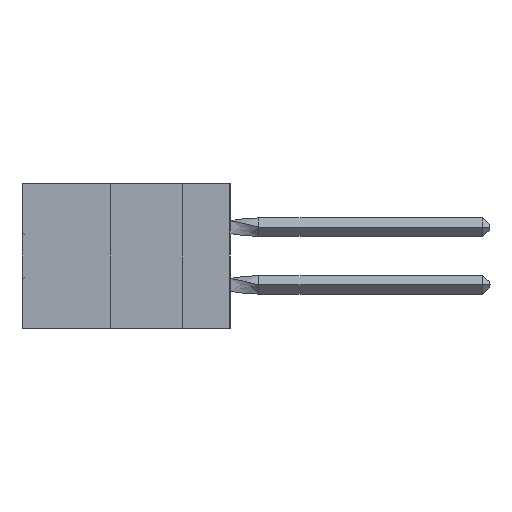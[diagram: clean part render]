
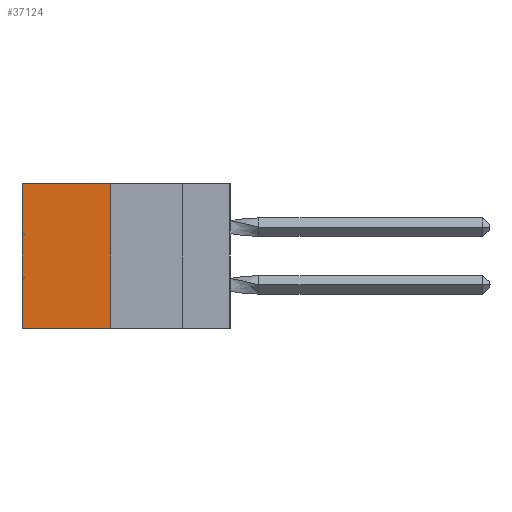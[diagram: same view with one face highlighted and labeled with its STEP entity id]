
A CAD part, left-side view. The second image highlights one B-rep face of the part: STEP entity #37124.
In plain terms, the highlighted planar face has unit normal (-1, 0, 0).
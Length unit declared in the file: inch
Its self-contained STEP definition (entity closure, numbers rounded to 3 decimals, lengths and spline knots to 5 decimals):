
#1311 = DIRECTION ( 'NONE',  ( 0., 0., -1. ) ) ;
#5220 = VERTEX_POINT ( 'NONE', #35647 ) ;
#5736 = FACE_OUTER_BOUND ( 'NONE', #34759, .T. ) ;
#5968 = ORIENTED_EDGE ( 'NONE', *, *, #28280, .T. ) ;
#6668 = VERTEX_POINT ( 'NONE', #11920 ) ;
#7921 = CARTESIAN_POINT ( 'NONE',  ( 0.305, 0.413, 0. ) ) ;
#8298 = EDGE_CURVE ( 'NONE', #5220, #6668, #28618, .T. ) ;
#9250 = DIRECTION ( 'NONE',  ( 0., 1., 0. ) ) ;
#10752 = VERTEX_POINT ( 'NONE', #39555 ) ;
#11899 = CARTESIAN_POINT ( 'NONE',  ( 0.305, 0.413, -0.5 ) ) ;
#11920 = CARTESIAN_POINT ( 'NONE',  ( 0.305, 0.413, -0.5 ) ) ;
#13196 = ORIENTED_EDGE ( 'NONE', *, *, #34501, .T. ) ;
#16130 = VECTOR ( 'NONE', #29575, 39.37008 ) ;
#17137 = EDGE_CURVE ( 'NONE', #6668, #10752, #24407, .T. ) ;
#18140 = VECTOR ( 'NONE', #28593, 39.37008 ) ;
#20359 = DIRECTION ( 'NONE',  ( 0., 1., 0. ) ) ;
#21467 = CARTESIAN_POINT ( 'NONE',  ( 0.305, 0.72, -0.5 ) ) ;
#22289 = AXIS2_PLACEMENT_3D ( 'NONE', #51419, #51596, #1311 ) ;
#23508 = VECTOR ( 'NONE', #20359, 39.37008 ) ;
#23637 = ORIENTED_EDGE ( 'NONE', *, *, #17137, .F. ) ;
#24407 = LINE ( 'NONE', #46908, #51894 ) ;
#28280 = EDGE_CURVE ( 'NONE', #5220, #39787, #35291, .T. ) ;
#28593 = DIRECTION ( 'NONE',  ( 0., 0., -1. ) ) ;
#28618 = LINE ( 'NONE', #11899, #18140 ) ;
#29575 = DIRECTION ( 'NONE',  ( 0., 0., -1. ) ) ;
#34248 = PLANE ( 'NONE',  #22289 ) ;
#34501 = EDGE_CURVE ( 'NONE', #39787, #10752, #50161, .T. ) ;
#34759 = EDGE_LOOP ( 'NONE', ( #13196, #23637, #35723, #5968 ) ) ;
#35291 = LINE ( 'NONE', #7921, #23508 ) ;
#35647 = CARTESIAN_POINT ( 'NONE',  ( 0.305, 0.413, 0. ) ) ;
#35723 = ORIENTED_EDGE ( 'NONE', *, *, #8298, .F. ) ;
#37124 = ADVANCED_FACE ( 'NONE', ( #5736 ), #34248, .F. ) ;
#39555 = CARTESIAN_POINT ( 'NONE',  ( 0.305, 0.72, -0.5 ) ) ;
#39787 = VERTEX_POINT ( 'NONE', #52205 ) ;
#46908 = CARTESIAN_POINT ( 'NONE',  ( 0.305, 0.413, -0.5 ) ) ;
#50161 = LINE ( 'NONE', #21467, #16130 ) ;
#51419 = CARTESIAN_POINT ( 'NONE',  ( 0.305, 0.413, -0.5 ) ) ;
#51596 = DIRECTION ( 'NONE',  ( 1., 0., 0. ) ) ;
#51894 = VECTOR ( 'NONE', #9250, 39.37008 ) ;
#52205 = CARTESIAN_POINT ( 'NONE',  ( 0.305, 0.72, 0. ) ) ;
